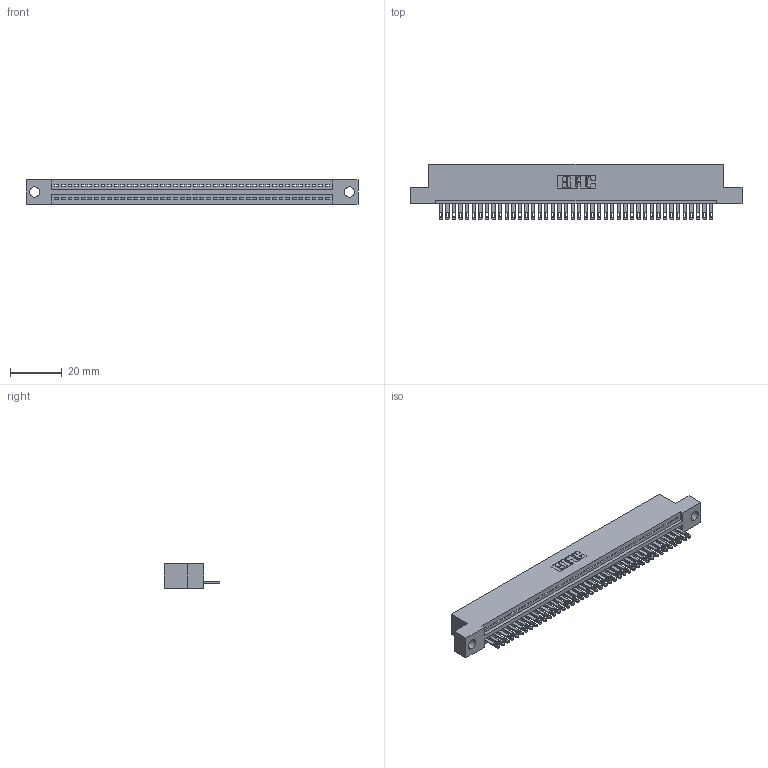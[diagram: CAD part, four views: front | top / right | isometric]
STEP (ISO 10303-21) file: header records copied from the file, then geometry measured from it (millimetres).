
FILE_DESCRIPTION (( 'STEP AP203' ), '1' );
FILE_NAME ('895-042-500-104.STEP', '2020-09-27T00:54:09', ( '' ), ( '' ), 'SwSTEP 2.0', 'SolidWorks 2020', '' );
FILE_SCHEMA (( 'CONFIG_CONTROL_DESIGN' ));
Length unit declared in the file: inch
Products named in the file (3): 895-042-500-104; 345-292-001_345-293-100; 845 Part_Flush Mounting Lugs - 0.156 Dia-TH
Assembly tree (43 placements, depth 2):
  895-042-500-104
    845 Part_Flush Mounting Lugs - 0.156 Dia-TH
    345-292-001_345-293-100  x42
Bounding box: 127.89 x 21.51 x 9.4 mm (x, y, z)
Volume: 12085.2 mm3; surface area: 15963.2 mm2
Topology: 43 solids, 43 shells, 2394 faces, 7397 edges, 4930 vertices
Faces by surface type: plane 1508, cylinder 886
Entity records: 31543 total; most frequent: CARTESIAN_POINT 5470, ORIENTED_EDGE 5446, DIRECTION 4779, EDGE_CURVE 2723, VECTOR 2419, LINE 2419, VERTEX_POINT 1814, AXIS2_PLACEMENT_3D 1180
